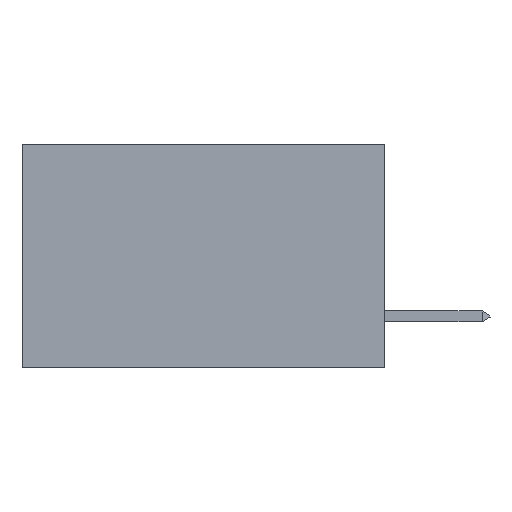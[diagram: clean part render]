
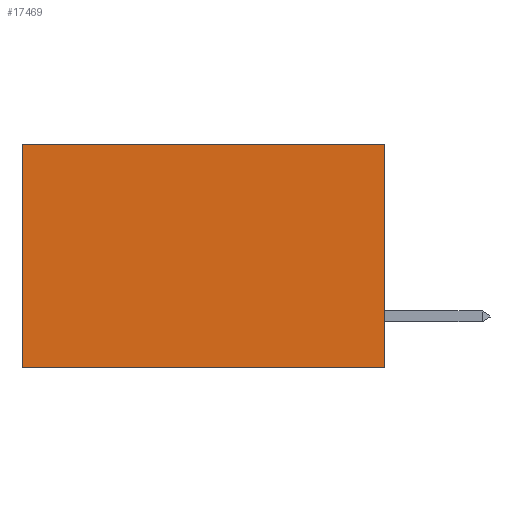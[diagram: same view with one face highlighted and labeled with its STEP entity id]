
A CAD part, left-side view. The second image highlights one B-rep face of the part: STEP entity #17469.
In plain terms, the highlighted planar face has unit normal (-1, 0, 0).
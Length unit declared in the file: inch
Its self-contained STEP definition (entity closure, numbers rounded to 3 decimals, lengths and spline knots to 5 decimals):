
#217 = EDGE_LOOP ( 'NONE', ( #14820, #19636, #19296, #18294 ) ) ;
#305 = EDGE_CURVE ( 'NONE', #25928, #16970, #8269, .T. ) ;
#458 = CARTESIAN_POINT ( 'NONE',  ( 0.2875, 0., -0.37 ) ) ;
#485 = VECTOR ( 'NONE', #15269, 39.37008 ) ;
#1495 = VECTOR ( 'NONE', #24178, 39.37008 ) ;
#2314 = VERTEX_POINT ( 'NONE', #25324 ) ;
#2408 = LINE ( 'NONE', #8200, #2731 ) ;
#2731 = VECTOR ( 'NONE', #12613, 39.37008 ) ;
#2948 = CARTESIAN_POINT ( 'NONE',  ( 0.2875, 0., 0. ) ) ;
#3330 = CARTESIAN_POINT ( 'NONE',  ( 0.2875, 0., 0. ) ) ;
#4156 = AXIS2_PLACEMENT_3D ( 'NONE', #3330, #7263, #26816 ) ;
#4847 = DIRECTION ( 'NONE',  ( 0., 0., -1. ) ) ;
#5389 = EDGE_CURVE ( 'NONE', #22023, #25928, #16243, .T. ) ;
#5989 = CARTESIAN_POINT ( 'NONE',  ( 0.2875, 0.6, -0.37 ) ) ;
#6476 = CARTESIAN_POINT ( 'NONE',  ( 0.2875, 0., 0. ) ) ;
#6950 = VECTOR ( 'NONE', #4847, 39.37008 ) ;
#7263 = DIRECTION ( 'NONE',  ( 1., 0., 0. ) ) ;
#8200 = CARTESIAN_POINT ( 'NONE',  ( 0.2875, 0., 0. ) ) ;
#8269 = LINE ( 'NONE', #13319, #6950 ) ;
#10217 = EDGE_CURVE ( 'NONE', #2314, #16970, #21246, .T. ) ;
#12578 = CARTESIAN_POINT ( 'NONE',  ( 0.2875, 0.6, 0. ) ) ;
#12613 = DIRECTION ( 'NONE',  ( 0., 0., -1. ) ) ;
#13319 = CARTESIAN_POINT ( 'NONE',  ( 0.2875, 0.6, 0. ) ) ;
#14820 = ORIENTED_EDGE ( 'NONE', *, *, #305, .T. ) ;
#15269 = DIRECTION ( 'NONE',  ( 0., 1., 0. ) ) ;
#16243 = LINE ( 'NONE', #2948, #1495 ) ;
#16970 = VERTEX_POINT ( 'NONE', #5989 ) ;
#17469 = ADVANCED_FACE ( 'NONE', ( #25817 ), #22297, .F. ) ;
#18294 = ORIENTED_EDGE ( 'NONE', *, *, #5389, .T. ) ;
#19296 = ORIENTED_EDGE ( 'NONE', *, *, #24132, .F. ) ;
#19636 = ORIENTED_EDGE ( 'NONE', *, *, #10217, .F. ) ;
#21246 = LINE ( 'NONE', #458, #485 ) ;
#22023 = VERTEX_POINT ( 'NONE', #6476 ) ;
#22297 = PLANE ( 'NONE',  #4156 ) ;
#24132 = EDGE_CURVE ( 'NONE', #22023, #2314, #2408, .T. ) ;
#24178 = DIRECTION ( 'NONE',  ( 0., 1., 0. ) ) ;
#25324 = CARTESIAN_POINT ( 'NONE',  ( 0.2875, 0., -0.37 ) ) ;
#25817 = FACE_OUTER_BOUND ( 'NONE', #217, .T. ) ;
#25928 = VERTEX_POINT ( 'NONE', #12578 ) ;
#26816 = DIRECTION ( 'NONE',  ( 0., 0., -1. ) ) ;
